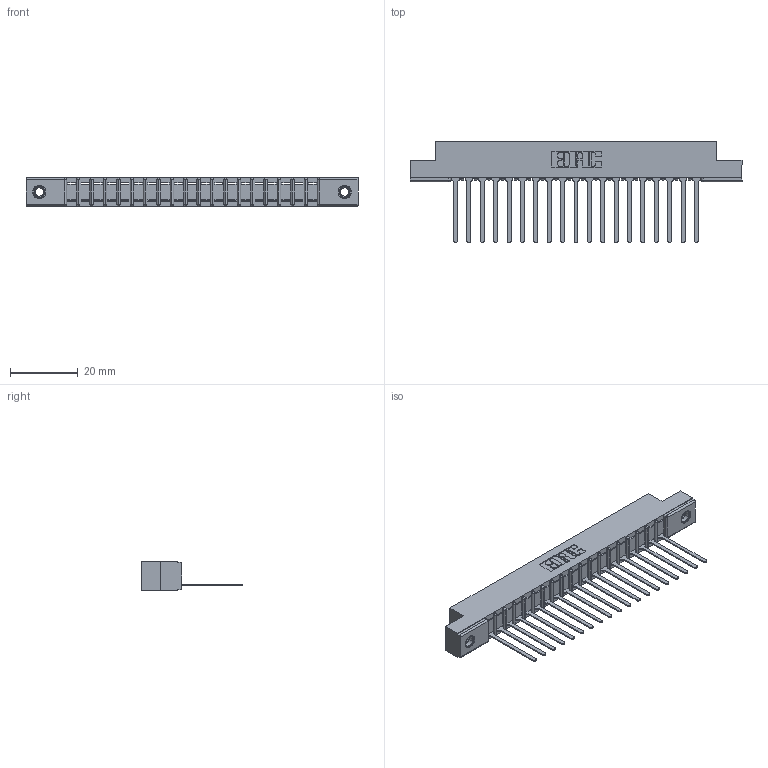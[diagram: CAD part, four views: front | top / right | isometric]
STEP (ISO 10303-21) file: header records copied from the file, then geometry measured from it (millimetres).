
FILE_DESCRIPTION (( 'STEP AP203' ), '1' );
FILE_NAME ('357-019-545-107.STEP', '2019-09-13T22:45:49', ( '' ), ( '' ), 'SwSTEP 2.0', 'SolidWorks 2016', '' );
FILE_SCHEMA (( 'CONFIG_CONTROL_DESIGN' ));
Length unit declared in the file: inch
Products named in the file (4): 357-019-545-107; 345-250-001_345-250-005-103; 307-290-001_545; 307 Part_.156 Dia Mounting Holes
Assembly tree (22 placements, depth 2):
  357-019-545-107
    307 Part_.156 Dia Mounting Holes
    307-290-001_545  x19
    345-250-001_345-250-005-103  x2
Bounding box: 98.3 x 30 x 8.71 mm (x, y, z)
Volume: 6277.5 mm3; surface area: 10127.6 mm2
Topology: 22 solids, 22 shells, 1262 faces, 3537 edges, 2270 vertices
Faces by surface type: plane 805, cylinder 401, sphere 40, cone 12, torus 4
Entity records: 20277 total; most frequent: CARTESIAN_POINT 3387, ORIENTED_EDGE 3366, DIRECTION 3317, EDGE_CURVE 1683, VECTOR 1281, LINE 1281, VERTEX_POINT 1088, AXIS2_PLACEMENT_3D 1018
